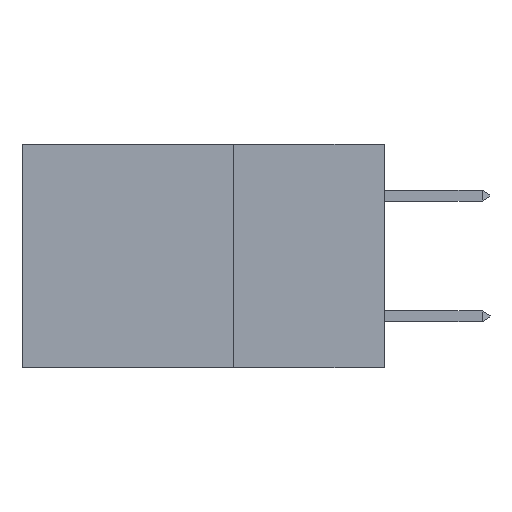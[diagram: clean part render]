
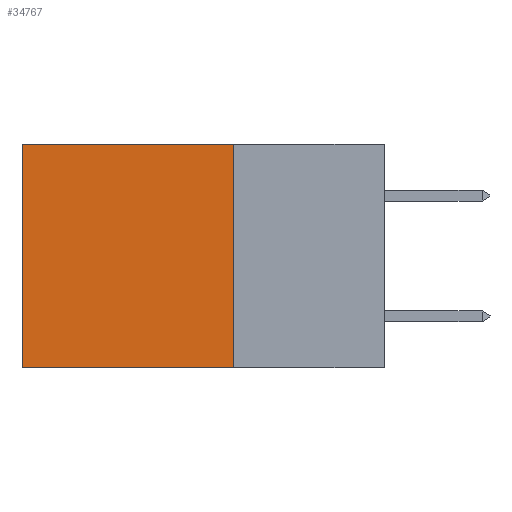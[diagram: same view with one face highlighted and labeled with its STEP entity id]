
A CAD part, left-side view. The second image highlights one B-rep face of the part: STEP entity #34767.
In plain terms, the highlighted planar face has unit normal (-1, 0, 0).
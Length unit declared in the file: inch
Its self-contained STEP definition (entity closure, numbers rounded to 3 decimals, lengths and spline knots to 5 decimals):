
#207 = DIRECTION ( 'NONE',  ( 1., 0., 0. ) ) ;
#2588 = VECTOR ( 'NONE', #11592, 39.37008 ) ;
#3666 = LINE ( 'NONE', #14593, #10388 ) ;
#4221 = CARTESIAN_POINT ( 'NONE',  ( 0.2875, 0.25, 0. ) ) ;
#5752 = FACE_OUTER_BOUND ( 'NONE', #35430, .T. ) ;
#6669 = EDGE_CURVE ( 'NONE', #18845, #16869, #12100, .T. ) ;
#9953 = VECTOR ( 'NONE', #23831, 39.37008 ) ;
#10388 = VECTOR ( 'NONE', #16759, 39.37008 ) ;
#11128 = DIRECTION ( 'NONE',  ( 0., 0., -1. ) ) ;
#11592 = DIRECTION ( 'NONE',  ( 0., 0., -1. ) ) ;
#12100 = LINE ( 'NONE', #4221, #35350 ) ;
#12343 = CARTESIAN_POINT ( 'NONE',  ( 0.2875, 0.25, 0. ) ) ;
#14109 = CARTESIAN_POINT ( 'NONE',  ( 0.2875, 0.6, 0. ) ) ;
#14593 = CARTESIAN_POINT ( 'NONE',  ( 0.2875, 0.25, -0.37 ) ) ;
#14667 = ORIENTED_EDGE ( 'NONE', *, *, #24504, .T. ) ;
#16359 = CARTESIAN_POINT ( 'NONE',  ( 0.2875, 0.25, -0.37 ) ) ;
#16690 = CARTESIAN_POINT ( 'NONE',  ( 0.2875, 0.25, 0. ) ) ;
#16759 = DIRECTION ( 'NONE',  ( 0., 1., 0. ) ) ;
#16869 = VERTEX_POINT ( 'NONE', #16359 ) ;
#17161 = LINE ( 'NONE', #14109, #2588 ) ;
#17539 = CARTESIAN_POINT ( 'NONE',  ( 0.2875, 0.6, -0.37 ) ) ;
#17677 = DIRECTION ( 'NONE',  ( 0., 0., -1. ) ) ;
#18845 = VERTEX_POINT ( 'NONE', #12343 ) ;
#19769 = EDGE_CURVE ( 'NONE', #16869, #21197, #3666, .T. ) ;
#20710 = ORIENTED_EDGE ( 'NONE', *, *, #31314, .T. ) ;
#21197 = VERTEX_POINT ( 'NONE', #17539 ) ;
#22135 = AXIS2_PLACEMENT_3D ( 'NONE', #16690, #207, #11128 ) ;
#23831 = DIRECTION ( 'NONE',  ( 0., 1., 0. ) ) ;
#24504 = EDGE_CURVE ( 'NONE', #18845, #26172, #29399, .T. ) ;
#24779 = PLANE ( 'NONE',  #22135 ) ;
#25434 = CARTESIAN_POINT ( 'NONE',  ( 0.2875, 0.6, 0. ) ) ;
#26172 = VERTEX_POINT ( 'NONE', #25434 ) ;
#26749 = ORIENTED_EDGE ( 'NONE', *, *, #6669, .F. ) ;
#27034 = ORIENTED_EDGE ( 'NONE', *, *, #19769, .F. ) ;
#29399 = LINE ( 'NONE', #34803, #9953 ) ;
#31314 = EDGE_CURVE ( 'NONE', #26172, #21197, #17161, .T. ) ;
#34767 = ADVANCED_FACE ( 'NONE', ( #5752 ), #24779, .F. ) ;
#34803 = CARTESIAN_POINT ( 'NONE',  ( 0.2875, 0.25, 0. ) ) ;
#35350 = VECTOR ( 'NONE', #17677, 39.37008 ) ;
#35430 = EDGE_LOOP ( 'NONE', ( #20710, #27034, #26749, #14667 ) ) ;
